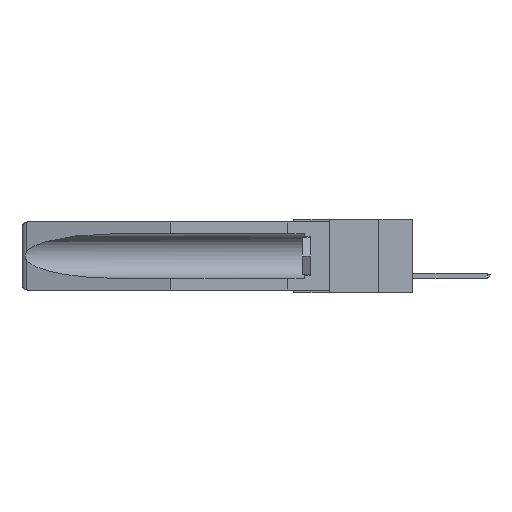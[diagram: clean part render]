
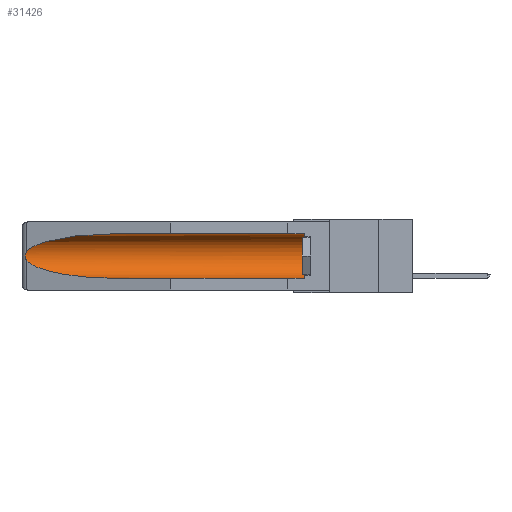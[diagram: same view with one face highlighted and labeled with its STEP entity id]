
A CAD part, left-side view. The second image highlights one B-rep face of the part: STEP entity #31426.
In plain terms, the highlighted cylindrical face has radius 2.857 mm (diameter 5.715 mm), a partial arc.
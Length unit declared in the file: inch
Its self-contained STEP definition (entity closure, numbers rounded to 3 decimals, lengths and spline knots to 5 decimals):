
#481 = CARTESIAN_POINT ( 'NONE',  ( 0.26537, 1.52718, -0.19328 ) ) ;
#1623 = CARTESIAN_POINT ( 'NONE',  ( 0.155, 0.126, -0.284 ) ) ;
#2467 = ORIENTED_EDGE ( 'NONE', *, *, #19005, .T. ) ;
#2811 = ORIENTED_EDGE ( 'NONE', *, *, #3912, .F. ) ;
#3425 = CARTESIAN_POINT ( 'NONE',  ( 0.2673, 1.53269, -0.17917 ) ) ;
#3912 = EDGE_CURVE ( 'NONE', #11560, #13533, #15363, .T. ) ;
#3952 = EDGE_CURVE ( 'NONE', #5075, #24467, #17445, .T. ) ;
#4620 = CARTESIAN_POINT ( 'NONE',  ( 0.155, -0.30754, -0.059 ) ) ;
#5075 = VERTEX_POINT ( 'NONE', #13667 ) ;
#5538 = CARTESIAN_POINT ( 'NONE',  ( 0.26597, 1.52961, -0.15275 ) ) ;
#5612 = CIRCLE ( 'NONE', #19797, 0.1125 ) ;
#5762 = CARTESIAN_POINT ( 'NONE',  ( 0.26655, 1.53094, -0.18657 ) ) ;
#5854 = CARTESIAN_POINT ( 'NONE',  ( 0.25451, 1.48313, -0.24835 ) ) ;
#7940 = CARTESIAN_POINT ( 'NONE',  ( 0.2675, 1.53308, -0.16763 ) ) ;
#8583 = CARTESIAN_POINT ( 'NONE',  ( 0.26537, 1.52718, -0.19328 ) ) ;
#8683 = VECTOR ( 'NONE', #13527, 39.37008 ) ;
#8903 = CYLINDRICAL_SURFACE ( 'NONE', #29164, 0.1125 ) ;
#9016 = CARTESIAN_POINT ( 'NONE',  ( 0.21114, 1.30732, -0.059 ) ) ;
#9582 = CARTESIAN_POINT ( 'NONE',  ( 0.26537, 1.52718, -0.19328 ) ) ;
#10301 = ORIENTED_EDGE ( 'NONE', *, *, #11390, .T. ) ;
#10398 = CARTESIAN_POINT ( 'NONE',  ( 0.26537, 1.52718, -0.14972 ) ) ;
#10666 = EDGE_LOOP ( 'NONE', ( #19396, #17271, #10301, #2811, #20700, #2467 ) ) ;
#11005 = VERTEX_POINT ( 'NONE', #24449 ) ;
#11229 = CARTESIAN_POINT ( 'NONE',  ( 0.21114, 1.30732, -0.284 ) ) ;
#11390 = EDGE_CURVE ( 'NONE', #30043, #13533, #14028, .T. ) ;
#11560 = VERTEX_POINT ( 'NONE', #1623 ) ;
#13527 = DIRECTION ( 'NONE',  ( 0., 1., 0. ) ) ;
#13533 = VERTEX_POINT ( 'NONE', #22853 ) ;
#13667 = CARTESIAN_POINT ( 'NONE',  ( 0.155, 1.07973, -0.059 ) ) ;
#14028 =( BOUNDED_CURVE ( )  B_SPLINE_CURVE ( 3, ( #8583, #5854, #11229, #21034 ),
 .UNSPECIFIED., .F., .F. ) 
 B_SPLINE_CURVE_WITH_KNOTS ( ( 4, 4 ),
 ( 0.1948, 1.5708 ),
 .UNSPECIFIED. ) 
 CURVE ( )  GEOMETRIC_REPRESENTATION_ITEM ( )  RATIONAL_B_SPLINE_CURVE ( ( 1., 0.848, 0.848, 1. ) ) 
 REPRESENTATION_ITEM ( '' )  );
#15363 = LINE ( 'NONE', #26097, #8683 ) ;
#15526 = CARTESIAN_POINT ( 'NONE',  ( 0.26654, 1.53092, -0.15636 ) ) ;
#17271 = ORIENTED_EDGE ( 'NONE', *, *, #23525, .T. ) ;
#17445 =( BOUNDED_CURVE ( )  B_SPLINE_CURVE ( 3, ( #21777, #9016, #21988, #19148 ),
 .UNSPECIFIED., .F., .F. ) 
 B_SPLINE_CURVE_WITH_KNOTS ( ( 4, 4 ),
 ( 4.71239, 6.08839 ),
 .UNSPECIFIED. ) 
 CURVE ( )  GEOMETRIC_REPRESENTATION_ITEM ( )  RATIONAL_B_SPLINE_CURVE ( ( 1., 0.848, 0.848, 1. ) ) 
 REPRESENTATION_ITEM ( '' )  );
#17849 = DIRECTION ( 'NONE',  ( 0., -1., 0. ) ) ;
#18074 = CARTESIAN_POINT ( 'NONE',  ( 0.2675, 1.53308, -0.17534 ) ) ;
#18412 = CARTESIAN_POINT ( 'NONE',  ( 0.26537, 1.52718, -0.14972 ) ) ;
#19005 = EDGE_CURVE ( 'NONE', #11005, #5075, #20559, .T. ) ;
#19148 = CARTESIAN_POINT ( 'NONE',  ( 0.26537, 1.52718, -0.14972 ) ) ;
#19396 = ORIENTED_EDGE ( 'NONE', *, *, #3952, .T. ) ;
#19778 = VECTOR ( 'NONE', #32210, 39.37008 ) ;
#19797 = AXIS2_PLACEMENT_3D ( 'NONE', #30306, #17849, #27785 ) ;
#20559 = LINE ( 'NONE', #4620, #19778 ) ;
#20595 = CARTESIAN_POINT ( 'NONE',  ( 0.26597, 1.5296, -0.19026 ) ) ;
#20700 = ORIENTED_EDGE ( 'NONE', *, *, #28245, .T. ) ;
#21034 = CARTESIAN_POINT ( 'NONE',  ( 0.155, 1.07973, -0.284 ) ) ;
#21777 = CARTESIAN_POINT ( 'NONE',  ( 0.155, 1.07973, -0.059 ) ) ;
#21988 = CARTESIAN_POINT ( 'NONE',  ( 0.25451, 1.48313, -0.09465 ) ) ;
#22853 = CARTESIAN_POINT ( 'NONE',  ( 0.155, 1.07973, -0.284 ) ) ;
#23109 = CARTESIAN_POINT ( 'NONE',  ( 0.2673, 1.5327, -0.16383 ) ) ;
#23503 = CARTESIAN_POINT ( 'NONE',  ( 0.155, -0.30754, -0.1715 ) ) ;
#23525 = EDGE_CURVE ( 'NONE', #24467, #30043, #32588, .T. ) ;
#23601 = DIRECTION ( 'NONE',  ( 0., 1., 0. ) ) ;
#24449 = CARTESIAN_POINT ( 'NONE',  ( 0.155, 0.126, -0.059 ) ) ;
#24467 = VERTEX_POINT ( 'NONE', #10398 ) ;
#26097 = CARTESIAN_POINT ( 'NONE',  ( 0.155, -0.30754, -0.284 ) ) ;
#27785 = DIRECTION ( 'NONE',  ( 0., 0., 1. ) ) ;
#28225 = FACE_OUTER_BOUND ( 'NONE', #10666, .T. ) ;
#28245 = EDGE_CURVE ( 'NONE', #11560, #11005, #5612, .T. ) ;
#29164 = AXIS2_PLACEMENT_3D ( 'NONE', #23503, #23601, #31214 ) ;
#30043 = VERTEX_POINT ( 'NONE', #9582 ) ;
#30306 = CARTESIAN_POINT ( 'NONE',  ( 0.155, 0.126, -0.1715 ) ) ;
#31214 = DIRECTION ( 'NONE',  ( 0., 0., 1. ) ) ;
#31426 = ADVANCED_FACE ( 'NONE', ( #28225 ), #8903, .F. ) ;
#32210 = DIRECTION ( 'NONE',  ( 0., 1., 0. ) ) ;
#32588 = B_SPLINE_CURVE_WITH_KNOTS ( 'NONE', 3,
 ( #18412, #5538, #15526, #23109, #7940, #18074, #3425, #5762, #20595, #481 ),
 .UNSPECIFIED., .F., .F.,
 ( 4, 2, 2, 2, 4 ),
 ( 0., 0.00029, 0.00058, 0.00087, 0.00117 ),
 .UNSPECIFIED. ) ;
